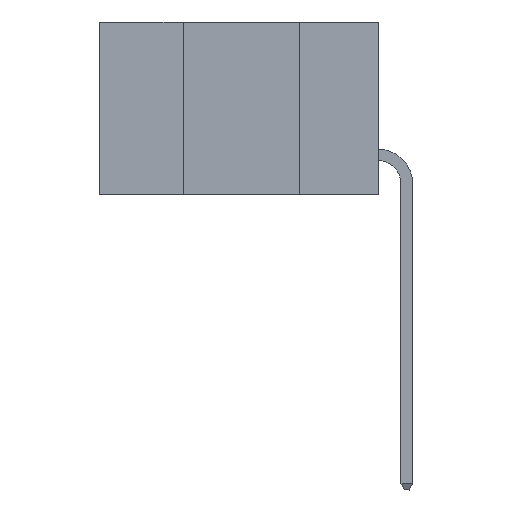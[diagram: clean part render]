
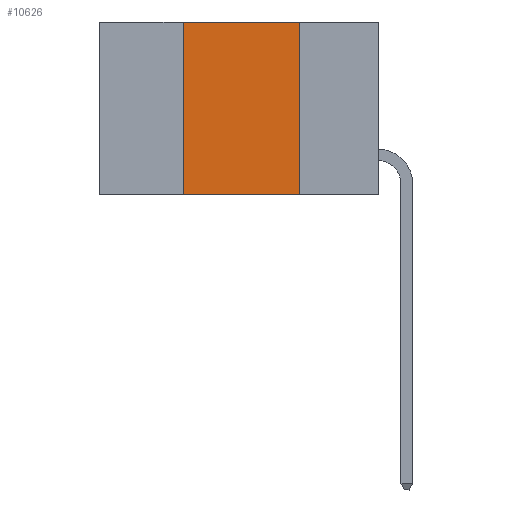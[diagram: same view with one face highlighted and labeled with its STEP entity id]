
A CAD part, left-side view. The second image highlights one B-rep face of the part: STEP entity #10626.
In plain terms, the highlighted planar face has unit normal (-1, 0, 0).
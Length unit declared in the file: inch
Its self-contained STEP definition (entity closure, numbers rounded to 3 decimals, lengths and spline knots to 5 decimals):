
#204 = CARTESIAN_POINT ( 'NONE',  ( 0., 0.6, -0.37 ) ) ;
#1206 = CARTESIAN_POINT ( 'NONE',  ( 0., 0.17, -0.37 ) ) ;
#1345 = LINE ( 'NONE', #204, #8179 ) ;
#1615 = DIRECTION ( 'NONE',  ( 0., -1., 0. ) ) ;
#1651 = DIRECTION ( 'NONE',  ( 0., 0., -1. ) ) ;
#2234 = VERTEX_POINT ( 'NONE', #17581 ) ;
#2504 = LINE ( 'NONE', #8704, #6115 ) ;
#3128 = DIRECTION ( 'NONE',  ( 0., -1., 0. ) ) ;
#3302 = ORIENTED_EDGE ( 'NONE', *, *, #9265, .F. ) ;
#3846 = ORIENTED_EDGE ( 'NONE', *, *, #15585, .F. ) ;
#3961 = CARTESIAN_POINT ( 'NONE',  ( 0., 0.17, 0. ) ) ;
#4550 = VERTEX_POINT ( 'NONE', #1206 ) ;
#5208 = ORIENTED_EDGE ( 'NONE', *, *, #17259, .T. ) ;
#5324 = EDGE_CURVE ( 'NONE', #16814, #13719, #17049, .T. ) ;
#5761 = ORIENTED_EDGE ( 'NONE', *, *, #5324, .F. ) ;
#6115 = VECTOR ( 'NONE', #8763, 39.37008 ) ;
#7531 = FACE_OUTER_BOUND ( 'NONE', #14533, .T. ) ;
#8179 = VECTOR ( 'NONE', #1615, 39.37008 ) ;
#8444 = PLANE ( 'NONE',  #8556 ) ;
#8539 = CARTESIAN_POINT ( 'NONE',  ( 0., 0.6, 0. ) ) ;
#8556 = AXIS2_PLACEMENT_3D ( 'NONE', #16790, #9822, #1651 ) ;
#8704 = CARTESIAN_POINT ( 'NONE',  ( 0., 0.17, 0. ) ) ;
#8763 = DIRECTION ( 'NONE',  ( 0., 0., -1. ) ) ;
#9265 = EDGE_CURVE ( 'NONE', #2234, #16814, #13021, .T. ) ;
#9822 = DIRECTION ( 'NONE',  ( 1., 0., 0. ) ) ;
#10626 = ADVANCED_FACE ( 'NONE', ( #7531 ), #8444, .F. ) ;
#11140 = DIRECTION ( 'NONE',  ( 0., 0., 1. ) ) ;
#12571 = VECTOR ( 'NONE', #11140, 39.37008 ) ;
#13021 = LINE ( 'NONE', #15351, #12571 ) ;
#13338 = VECTOR ( 'NONE', #3128, 39.37008 ) ;
#13719 = VERTEX_POINT ( 'NONE', #3961 ) ;
#14533 = EDGE_LOOP ( 'NONE', ( #3846, #5761, #3302, #5208 ) ) ;
#15351 = CARTESIAN_POINT ( 'NONE',  ( 0., 0.42, 0. ) ) ;
#15585 = EDGE_CURVE ( 'NONE', #13719, #4550, #2504, .T. ) ;
#15595 = CARTESIAN_POINT ( 'NONE',  ( 0., 0.42, 0. ) ) ;
#16790 = CARTESIAN_POINT ( 'NONE',  ( 0., 0.6, 0. ) ) ;
#16814 = VERTEX_POINT ( 'NONE', #15595 ) ;
#17049 = LINE ( 'NONE', #8539, #13338 ) ;
#17259 = EDGE_CURVE ( 'NONE', #2234, #4550, #1345, .T. ) ;
#17581 = CARTESIAN_POINT ( 'NONE',  ( 0., 0.42, -0.37 ) ) ;
